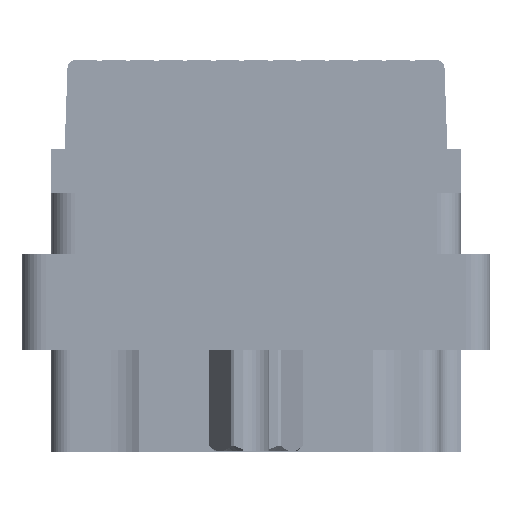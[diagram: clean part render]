
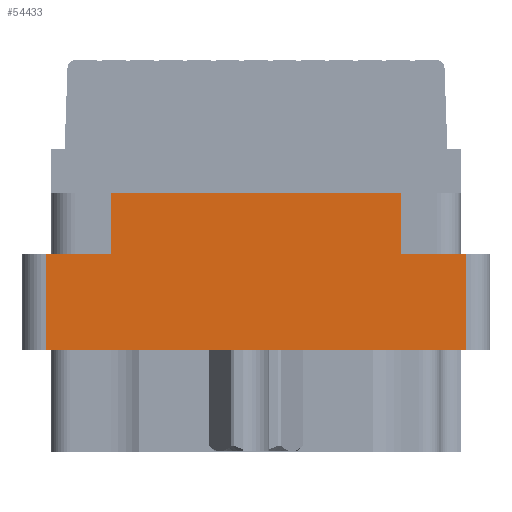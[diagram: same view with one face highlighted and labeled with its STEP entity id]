
A CAD part, left-side view. The second image highlights one B-rep face of the part: STEP entity #54433.
In plain terms, the highlighted planar face has unit normal (-1, 0, 0).
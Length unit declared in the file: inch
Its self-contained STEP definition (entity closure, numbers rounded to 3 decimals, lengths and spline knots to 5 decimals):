
#280 = CARTESIAN_POINT ( 'NONE',  ( -1.359, -0.617, -0.798 ) ) ;
#409 = CARTESIAN_POINT ( 'NONE',  ( -1.359, 0., -0.529 ) ) ;
#3506 = EDGE_CURVE ( 'NONE', #65538, #52708, #83770, .T. ) ;
#6015 = CARTESIAN_POINT ( 'NONE',  ( -1.359, 0.555, -0.529 ) ) ;
#7299 = LINE ( 'NONE', #33088, #50507 ) ;
#7994 = CARTESIAN_POINT ( 'NONE',  ( -1.359, 0.617, -0.117 ) ) ;
#11603 = DIRECTION ( 'NONE',  ( 0., 0., 1. ) ) ;
#12023 = CARTESIAN_POINT ( 'NONE',  ( -1.359, 0.3825, -0.277 ) ) ;
#12543 = DIRECTION ( 'NONE',  ( -1., 0., 0. ) ) ;
#12823 = VERTEX_POINT ( 'NONE', #81385 ) ;
#13488 = VECTOR ( 'NONE', #70711, 39.37008 ) ;
#13824 = CARTESIAN_POINT ( 'NONE',  ( -1.359, -0.3825, -0.277 ) ) ;
#16581 = CARTESIAN_POINT ( 'NONE',  ( -1.359, 0.3825, -0.117 ) ) ;
#16809 = CARTESIAN_POINT ( 'NONE',  ( -1.359, 0.555, -0.798 ) ) ;
#17180 = DIRECTION ( 'NONE',  ( 0., -1., 0. ) ) ;
#18799 = VECTOR ( 'NONE', #39663, 39.37008 ) ;
#21496 = LINE ( 'NONE', #7994, #81165 ) ;
#26207 = DIRECTION ( 'NONE',  ( 0., 1., 0. ) ) ;
#29090 = DIRECTION ( 'NONE',  ( 0., 0., -1. ) ) ;
#29509 = LINE ( 'NONE', #16809, #58252 ) ;
#31143 = CARTESIAN_POINT ( 'NONE',  ( -1.359, 0., -0.277 ) ) ;
#32539 = LINE ( 'NONE', #50802, #13488 ) ;
#32954 = EDGE_LOOP ( 'NONE', ( #50602, #71889, #60906, #56354, #54416, #74555, #55172, #52477 ) ) ;
#33088 = CARTESIAN_POINT ( 'NONE',  ( -1.359, -0.555, -0.798 ) ) ;
#34499 = CARTESIAN_POINT ( 'NONE',  ( -1.359, -0.555, -0.529 ) ) ;
#35373 = AXIS2_PLACEMENT_3D ( 'NONE', #280, #12543, #51541 ) ;
#35409 = EDGE_CURVE ( 'NONE', #43894, #80075, #71894, .T. ) ;
#35862 = PLANE ( 'NONE',  #35373 ) ;
#37637 = EDGE_CURVE ( 'NONE', #12823, #57800, #38677, .T. ) ;
#38069 = EDGE_CURVE ( 'NONE', #43894, #60400, #32539, .T. ) ;
#38171 = EDGE_CURVE ( 'NONE', #57800, #80075, #21496, .T. ) ;
#38339 = EDGE_CURVE ( 'NONE', #67390, #52708, #29509, .T. ) ;
#38677 = LINE ( 'NONE', #12023, #68879 ) ;
#39663 = DIRECTION ( 'NONE',  ( 0., 0., 1. ) ) ;
#40285 = VECTOR ( 'NONE', #26207, 39.37008 ) ;
#40522 = VECTOR ( 'NONE', #17180, 39.37008 ) ;
#43894 = VERTEX_POINT ( 'NONE', #57415 ) ;
#47370 = DIRECTION ( 'NONE',  ( 0., -1., 0. ) ) ;
#50507 = VECTOR ( 'NONE', #52630, 39.37008 ) ;
#50602 = ORIENTED_EDGE ( 'NONE', *, *, #73219, .F. ) ;
#50802 = CARTESIAN_POINT ( 'NONE',  ( -1.359, 0., -0.277 ) ) ;
#51541 = DIRECTION ( 'NONE',  ( 0., 0., 1. ) ) ;
#52477 = ORIENTED_EDGE ( 'NONE', *, *, #37637, .F. ) ;
#52630 = DIRECTION ( 'NONE',  ( 0., 0., 1. ) ) ;
#52708 = VERTEX_POINT ( 'NONE', #6015 ) ;
#54416 = ORIENTED_EDGE ( 'NONE', *, *, #38069, .F. ) ;
#54433 = ADVANCED_FACE ( 'NONE', ( #68085 ), #35862, .T. ) ;
#55172 = ORIENTED_EDGE ( 'NONE', *, *, #38171, .F. ) ;
#56354 = ORIENTED_EDGE ( 'NONE', *, *, #78207, .T. ) ;
#57415 = CARTESIAN_POINT ( 'NONE',  ( -1.359, -0.3825, -0.277 ) ) ;
#57800 = VERTEX_POINT ( 'NONE', #16581 ) ;
#58252 = VECTOR ( 'NONE', #29090, 39.37008 ) ;
#60400 = VERTEX_POINT ( 'NONE', #67542 ) ;
#60906 = ORIENTED_EDGE ( 'NONE', *, *, #3506, .F. ) ;
#65538 = VERTEX_POINT ( 'NONE', #34499 ) ;
#67390 = VERTEX_POINT ( 'NONE', #83073 ) ;
#67542 = CARTESIAN_POINT ( 'NONE',  ( -1.359, -0.555, -0.277 ) ) ;
#67751 = CARTESIAN_POINT ( 'NONE',  ( -1.359, -0.3825, -0.117 ) ) ;
#68085 = FACE_OUTER_BOUND ( 'NONE', #32954, .T. ) ;
#68879 = VECTOR ( 'NONE', #11603, 39.37008 ) ;
#70711 = DIRECTION ( 'NONE',  ( 0., -1., 0. ) ) ;
#71889 = ORIENTED_EDGE ( 'NONE', *, *, #38339, .T. ) ;
#71894 = LINE ( 'NONE', #13824, #18799 ) ;
#73219 = EDGE_CURVE ( 'NONE', #67390, #12823, #80355, .T. ) ;
#74555 = ORIENTED_EDGE ( 'NONE', *, *, #35409, .T. ) ;
#78207 = EDGE_CURVE ( 'NONE', #65538, #60400, #7299, .T. ) ;
#80075 = VERTEX_POINT ( 'NONE', #67751 ) ;
#80355 = LINE ( 'NONE', #31143, #40522 ) ;
#81165 = VECTOR ( 'NONE', #47370, 39.37008 ) ;
#81385 = CARTESIAN_POINT ( 'NONE',  ( -1.359, 0.3825, -0.277 ) ) ;
#83073 = CARTESIAN_POINT ( 'NONE',  ( -1.359, 0.555, -0.277 ) ) ;
#83770 = LINE ( 'NONE', #409, #40285 ) ;
